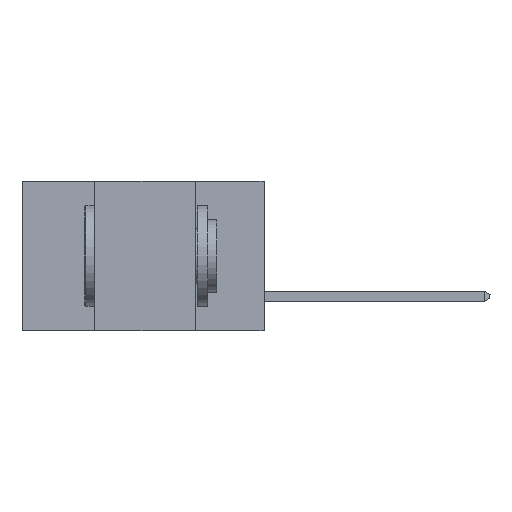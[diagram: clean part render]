
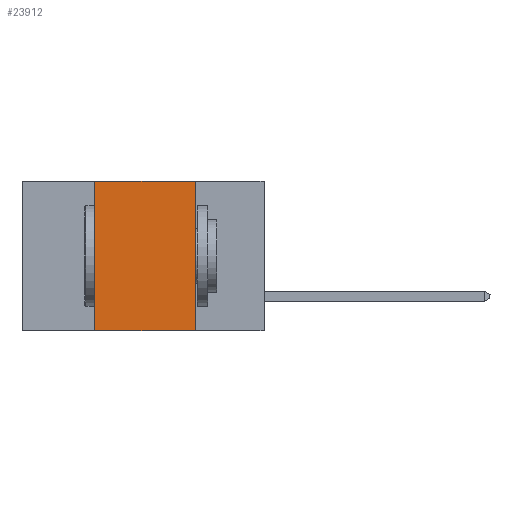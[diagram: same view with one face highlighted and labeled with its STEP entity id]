
A CAD part, left-side view. The second image highlights one B-rep face of the part: STEP entity #23912.
In plain terms, the highlighted planar face has unit normal (-1, 0, 0).
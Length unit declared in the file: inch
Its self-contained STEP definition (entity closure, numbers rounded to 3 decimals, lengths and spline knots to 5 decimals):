
#157 = PLANE ( 'NONE',  #20919 ) ;
#770 = EDGE_CURVE ( 'NONE', #6713, #20448, #2104, .T. ) ;
#2104 = LINE ( 'NONE', #5710, #13224 ) ;
#4628 = CARTESIAN_POINT ( 'NONE',  ( 0., 0.42, -0.37 ) ) ;
#4868 = LINE ( 'NONE', #22121, #23300 ) ;
#4978 = CARTESIAN_POINT ( 'NONE',  ( 0., 0.17, -0.37 ) ) ;
#5110 = DIRECTION ( 'NONE',  ( 0., -1., 0. ) ) ;
#5710 = CARTESIAN_POINT ( 'NONE',  ( 0., 0.6, -0.37 ) ) ;
#6097 = EDGE_CURVE ( 'NONE', #22319, #20448, #7895, .T. ) ;
#6713 = VERTEX_POINT ( 'NONE', #4628 ) ;
#7318 = ORIENTED_EDGE ( 'NONE', *, *, #6097, .F. ) ;
#7494 = EDGE_CURVE ( 'NONE', #6713, #13006, #17926, .T. ) ;
#7856 = DIRECTION ( 'NONE',  ( 0., 0., -1. ) ) ;
#7895 = LINE ( 'NONE', #11381, #11299 ) ;
#9687 = EDGE_LOOP ( 'NONE', ( #7318, #23939, #23495, #18864 ) ) ;
#10002 = CARTESIAN_POINT ( 'NONE',  ( 0., 0.17, 0. ) ) ;
#11299 = VECTOR ( 'NONE', #20806, 39.37008 ) ;
#11381 = CARTESIAN_POINT ( 'NONE',  ( 0., 0.17, -0.37 ) ) ;
#13006 = VERTEX_POINT ( 'NONE', #24451 ) ;
#13224 = VECTOR ( 'NONE', #14813, 39.37008 ) ;
#13680 = FACE_OUTER_BOUND ( 'NONE', #9687, .T. ) ;
#14813 = DIRECTION ( 'NONE',  ( 0., -1., 0. ) ) ;
#16073 = CARTESIAN_POINT ( 'NONE',  ( 0., 0.42, -0.37 ) ) ;
#16097 = VECTOR ( 'NONE', #21671, 39.37008 ) ;
#17926 = LINE ( 'NONE', #16073, #16097 ) ;
#18864 = ORIENTED_EDGE ( 'NONE', *, *, #770, .T. ) ;
#20448 = VERTEX_POINT ( 'NONE', #4978 ) ;
#20806 = DIRECTION ( 'NONE',  ( 0., 0., -1. ) ) ;
#20891 = DIRECTION ( 'NONE',  ( 1., 0., 0. ) ) ;
#20919 = AXIS2_PLACEMENT_3D ( 'NONE', #21022, #20891, #7856 ) ;
#21022 = CARTESIAN_POINT ( 'NONE',  ( 0., 0.6, 0. ) ) ;
#21671 = DIRECTION ( 'NONE',  ( 0., 0., 1. ) ) ;
#22121 = CARTESIAN_POINT ( 'NONE',  ( 0., 0.6, 0. ) ) ;
#22319 = VERTEX_POINT ( 'NONE', #10002 ) ;
#23300 = VECTOR ( 'NONE', #5110, 39.37008 ) ;
#23495 = ORIENTED_EDGE ( 'NONE', *, *, #7494, .F. ) ;
#23912 = ADVANCED_FACE ( 'NONE', ( #13680 ), #157, .F. ) ;
#23939 = ORIENTED_EDGE ( 'NONE', *, *, #24229, .F. ) ;
#24229 = EDGE_CURVE ( 'NONE', #13006, #22319, #4868, .T. ) ;
#24451 = CARTESIAN_POINT ( 'NONE',  ( 0., 0.42, 0. ) ) ;
